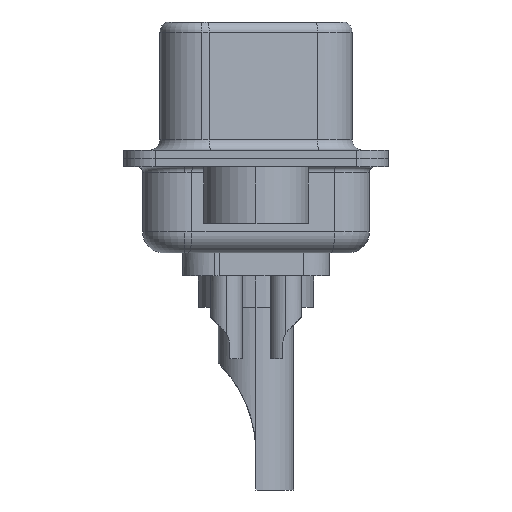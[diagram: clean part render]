
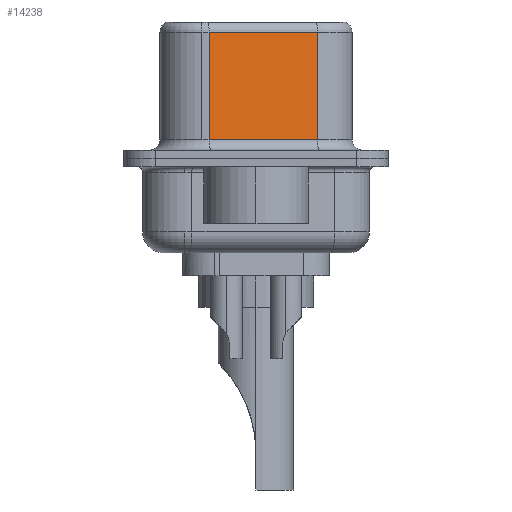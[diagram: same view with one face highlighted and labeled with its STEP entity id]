
A CAD part, left-side view. The second image highlights one B-rep face of the part: STEP entity #14238.
In plain terms, the highlighted planar face has unit normal (-0.985, -0.174, 0).
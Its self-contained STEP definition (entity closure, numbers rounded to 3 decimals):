
#6 = ORIENTED_EDGE ( 'NONE', *, *, #10991, .F. ) ;
#134 = LINE ( 'NONE', #4565, #3848 ) ;
#178 = CARTESIAN_POINT ( 'NONE',  ( 4.565, -2.927, 6.02 ) ) ;
#466 = VERTEX_POINT ( 'NONE', #550 ) ;
#550 = CARTESIAN_POINT ( 'NONE',  ( 4.565, -2.927, 6.02 ) ) ;
#1757 = DIRECTION ( 'NONE',  ( 0., 0., -1. ) ) ;
#1837 = EDGE_LOOP ( 'NONE', ( #6, #2774, #6006, #6761 ) ) ;
#2531 = CARTESIAN_POINT ( 'NONE',  ( 3.655, 2.233, 0.9 ) ) ;
#2774 = ORIENTED_EDGE ( 'NONE', *, *, #15220, .T. ) ;
#2896 = LINE ( 'NONE', #3154, #16712 ) ;
#2898 = EDGE_CURVE ( 'NONE', #9057, #16466, #15290, .T. ) ;
#3057 = LINE ( 'NONE', #178, #6399 ) ;
#3154 = CARTESIAN_POINT ( 'NONE',  ( 4.565, -2.927, 6.52 ) ) ;
#3848 = VECTOR ( 'NONE', #1757, 1000. ) ;
#4565 = CARTESIAN_POINT ( 'NONE',  ( 3.655, 2.233, 6.52 ) ) ;
#4658 = VECTOR ( 'NONE', #5733, 1000. ) ;
#5300 = CARTESIAN_POINT ( 'NONE',  ( 4.565, -2.927, 0.9 ) ) ;
#5733 = DIRECTION ( 'NONE',  ( 0.174, -0.985, 0. ) ) ;
#5902 = PLANE ( 'NONE',  #12290 ) ;
#6006 = ORIENTED_EDGE ( 'NONE', *, *, #7069, .T. ) ;
#6399 = VECTOR ( 'NONE', #9952, 1000. ) ;
#6709 = CARTESIAN_POINT ( 'NONE',  ( 4.565, -2.927, 0.9 ) ) ;
#6761 = ORIENTED_EDGE ( 'NONE', *, *, #2898, .T. ) ;
#7069 = EDGE_CURVE ( 'NONE', #10482, #9057, #134, .T. ) ;
#7264 = DIRECTION ( 'NONE',  ( -0.174, 0.985, 0. ) ) ;
#8571 = CARTESIAN_POINT ( 'NONE',  ( 4.565, -2.927, 6.52 ) ) ;
#9057 = VERTEX_POINT ( 'NONE', #2531 ) ;
#9952 = DIRECTION ( 'NONE',  ( -0.174, 0.985, 0. ) ) ;
#10023 = CARTESIAN_POINT ( 'NONE',  ( 3.655, 2.233, 6.02 ) ) ;
#10482 = VERTEX_POINT ( 'NONE', #10023 ) ;
#10991 = EDGE_CURVE ( 'NONE', #466, #16466, #2896, .T. ) ;
#12290 = AXIS2_PLACEMENT_3D ( 'NONE', #8571, #15097, #7264 ) ;
#14238 = ADVANCED_FACE ( 'NONE', ( #16264 ), #5902, .F. ) ;
#15097 = DIRECTION ( 'NONE',  ( 0.985, 0.174, 0. ) ) ;
#15220 = EDGE_CURVE ( 'NONE', #466, #10482, #3057, .T. ) ;
#15246 = DIRECTION ( 'NONE',  ( 0., 0., -1. ) ) ;
#15290 = LINE ( 'NONE', #6709, #4658 ) ;
#16264 = FACE_OUTER_BOUND ( 'NONE', #1837, .T. ) ;
#16466 = VERTEX_POINT ( 'NONE', #5300 ) ;
#16712 = VECTOR ( 'NONE', #15246, 1000. ) ;
